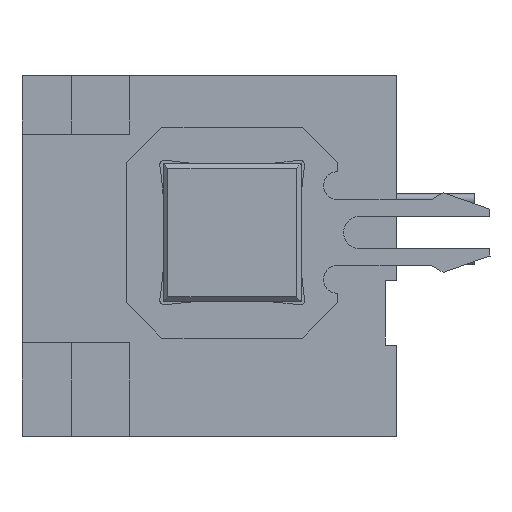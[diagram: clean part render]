
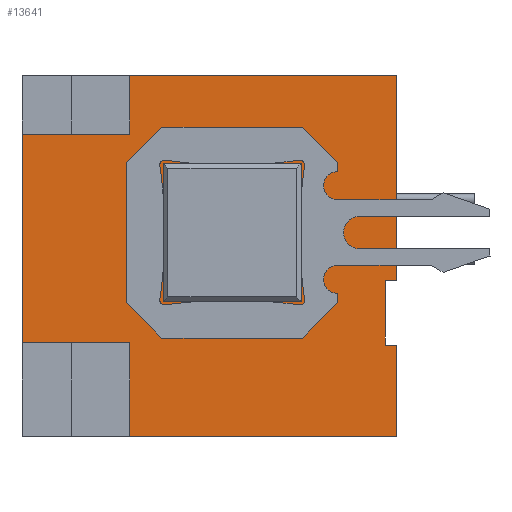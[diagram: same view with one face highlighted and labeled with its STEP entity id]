
A CAD part, left-side view. The second image highlights one B-rep face of the part: STEP entity #13641.
In plain terms, the highlighted planar face has unit normal (-1, 0, 0).
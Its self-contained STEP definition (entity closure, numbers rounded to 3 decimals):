
#40 = DIRECTION ( 'NONE',  ( 0., 0., 1. ) ) ;
#643 = DIRECTION ( 'NONE',  ( 0., 1., 0. ) ) ;
#648 = LINE ( 'NONE', #10963, #20650 ) ;
#688 = DIRECTION ( 'NONE',  ( 0., -1., 0. ) ) ;
#692 = CARTESIAN_POINT ( 'NONE',  ( -14.2, 1.975, 3.945 ) ) ;
#731 = VERTEX_POINT ( 'NONE', #20178 ) ;
#1031 = CARTESIAN_POINT ( 'NONE',  ( -14.2, -3.915, -1.945 ) ) ;
#1243 = CARTESIAN_POINT ( 'NONE',  ( -14.2, 3.4, -7.7 ) ) ;
#1359 = VERTEX_POINT ( 'NONE', #1243 ) ;
#1480 = ORIENTED_EDGE ( 'NONE', *, *, #5969, .F. ) ;
#1513 = VERTEX_POINT ( 'NONE', #15377 ) ;
#1740 = DIRECTION ( 'NONE',  ( 0., 0., 1. ) ) ;
#1865 = DIRECTION ( 'NONE',  ( 0., 0., 1. ) ) ;
#1890 = CARTESIAN_POINT ( 'NONE',  ( -14.2, 3.4, -3.7 ) ) ;
#2224 = DIRECTION ( 'NONE',  ( 0., 0., -1. ) ) ;
#2297 = VERTEX_POINT ( 'NONE', #26290 ) ;
#2396 = CARTESIAN_POINT ( 'NONE',  ( -14.2, -8., 0. ) ) ;
#2933 = LINE ( 'NONE', #2396, #24023 ) ;
#3200 = LINE ( 'NONE', #21412, #25618 ) ;
#3273 = DIRECTION ( 'NONE',  ( 0., 0., 1. ) ) ;
#3357 = LINE ( 'NONE', #13885, #6747 ) ;
#3377 = VECTOR ( 'NONE', #2224, 1000. ) ;
#3467 = EDGE_CURVE ( 'NONE', #19096, #731, #24400, .T. ) ;
#3474 = VECTOR ( 'NONE', #28197, 1000. ) ;
#3495 = LINE ( 'NONE', #22091, #16701 ) ;
#3871 = EDGE_LOOP ( 'NONE', ( #3902, #7708, #25490, #9734 ) ) ;
#3902 = ORIENTED_EDGE ( 'NONE', *, *, #3467, .T. ) ;
#4520 = CARTESIAN_POINT ( 'NONE',  ( -14.2, 1.975, 1. ) ) ;
#4812 = DIRECTION ( 'NONE',  ( 0., 1., 0. ) ) ;
#4821 = FACE_BOUND ( 'NONE', #3871, .T. ) ;
#5153 = EDGE_CURVE ( 'NONE', #24769, #12141, #3495, .T. ) ;
#5224 = VECTOR ( 'NONE', #17826, 1000. ) ;
#5384 = CARTESIAN_POINT ( 'NONE',  ( -14.2, -7.5, -1.05 ) ) ;
#5502 = CARTESIAN_POINT ( 'NONE',  ( -14.2, 3.4, 7.7 ) ) ;
#5545 = VERTEX_POINT ( 'NONE', #19291 ) ;
#5969 = EDGE_CURVE ( 'NONE', #5545, #22792, #13138, .T. ) ;
#6302 = CARTESIAN_POINT ( 'NONE',  ( -14.2, -3.915, 1. ) ) ;
#6424 = ORIENTED_EDGE ( 'NONE', *, *, #18494, .F. ) ;
#6539 = EDGE_CURVE ( 'NONE', #24769, #17950, #2933, .T. ) ;
#6632 = CARTESIAN_POINT ( 'NONE',  ( -14.2, -7.5, 0. ) ) ;
#6747 = VECTOR ( 'NONE', #3273, 1000. ) ;
#6896 = LINE ( 'NONE', #22305, #27308 ) ;
#7298 = DIRECTION ( 'NONE',  ( 0., 1., 0. ) ) ;
#7496 = LINE ( 'NONE', #9588, #24172 ) ;
#7708 = ORIENTED_EDGE ( 'NONE', *, *, #15140, .T. ) ;
#7783 = PLANE ( 'NONE',  #19110 ) ;
#7878 = CARTESIAN_POINT ( 'NONE',  ( -14.2, 8.32, 8.008 ) ) ;
#8138 = DIRECTION ( 'NONE',  ( 0., -1., 0. ) ) ;
#8441 = DIRECTION ( 'NONE',  ( 0., -1., 0. ) ) ;
#8472 = EDGE_CURVE ( 'NONE', #25409, #2297, #6896, .T. ) ;
#8482 = ORIENTED_EDGE ( 'NONE', *, *, #6539, .F. ) ;
#8525 = LINE ( 'NONE', #12983, #3474 ) ;
#8672 = VERTEX_POINT ( 'NONE', #5502 ) ;
#8795 = EDGE_CURVE ( 'NONE', #8672, #5545, #8525, .T. ) ;
#8842 = EDGE_LOOP ( 'NONE', ( #11366, #1480, #15389, #16690, #10026, #6424, #17616, #9783, #15792, #8482, #26615, #25506 ) ) ;
#9061 = DIRECTION ( 'NONE',  ( 0., 0., -1. ) ) ;
#9180 = EDGE_CURVE ( 'NONE', #1359, #25409, #23495, .T. ) ;
#9265 = CARTESIAN_POINT ( 'NONE',  ( -14.2, -7.75, -1.05 ) ) ;
#9357 = VECTOR ( 'NONE', #9061, 1000. ) ;
#9502 = VERTEX_POINT ( 'NONE', #692 ) ;
#9588 = CARTESIAN_POINT ( 'NONE',  ( -14.2, 0., 5.2 ) ) ;
#9734 = ORIENTED_EDGE ( 'NONE', *, *, #15179, .T. ) ;
#9783 = ORIENTED_EDGE ( 'NONE', *, *, #9180, .F. ) ;
#10026 = ORIENTED_EDGE ( 'NONE', *, *, #27849, .F. ) ;
#10293 = CARTESIAN_POINT ( 'NONE',  ( -14.2, -8., -1.05 ) ) ;
#10387 = EDGE_CURVE ( 'NONE', #1513, #8672, #648, .T. ) ;
#10758 = LINE ( 'NONE', #27767, #13491 ) ;
#10963 = CARTESIAN_POINT ( 'NONE',  ( -14.2, 3.4, 0. ) ) ;
#11241 = EDGE_CURVE ( 'NONE', #9502, #15343, #10758, .T. ) ;
#11366 = ORIENTED_EDGE ( 'NONE', *, *, #12251, .T. ) ;
#11656 = LINE ( 'NONE', #9265, #5224 ) ;
#12122 = LINE ( 'NONE', #6632, #23024 ) ;
#12141 = VERTEX_POINT ( 'NONE', #17726 ) ;
#12251 = EDGE_CURVE ( 'NONE', #21208, #22792, #11656, .T. ) ;
#12983 = CARTESIAN_POINT ( 'NONE',  ( -14.2, 0., 7.7 ) ) ;
#13138 = LINE ( 'NONE', #17811, #9357 ) ;
#13491 = VECTOR ( 'NONE', #8441, 1000. ) ;
#13641 = ADVANCED_FACE ( 'NONE', ( #4821, #23860 ), #7783, .F. ) ;
#13885 = CARTESIAN_POINT ( 'NONE',  ( -14.2, 8., 0. ) ) ;
#14332 = DIRECTION ( 'NONE',  ( 1., 0., 0. ) ) ;
#14651 = VECTOR ( 'NONE', #1740, 1000. ) ;
#15140 = EDGE_CURVE ( 'NONE', #731, #9502, #24761, .T. ) ;
#15179 = EDGE_CURVE ( 'NONE', #15343, #19096, #26135, .T. ) ;
#15343 = VERTEX_POINT ( 'NONE', #24912 ) ;
#15377 = CARTESIAN_POINT ( 'NONE',  ( -14.2, 3.4, 5.2 ) ) ;
#15389 = ORIENTED_EDGE ( 'NONE', *, *, #8795, .F. ) ;
#15792 = ORIENTED_EDGE ( 'NONE', *, *, #26132, .F. ) ;
#16265 = EDGE_CURVE ( 'NONE', #21208, #12141, #12122, .T. ) ;
#16690 = ORIENTED_EDGE ( 'NONE', *, *, #10387, .F. ) ;
#16701 = VECTOR ( 'NONE', #4812, 1000. ) ;
#17616 = ORIENTED_EDGE ( 'NONE', *, *, #8472, .F. ) ;
#17726 = CARTESIAN_POINT ( 'NONE',  ( -14.2, -7.5, -3.8 ) ) ;
#17811 = CARTESIAN_POINT ( 'NONE',  ( -14.2, -8., 0. ) ) ;
#17826 = DIRECTION ( 'NONE',  ( 0., -1., 0. ) ) ;
#17950 = VERTEX_POINT ( 'NONE', #20936 ) ;
#18494 = EDGE_CURVE ( 'NONE', #2297, #23355, #3357, .T. ) ;
#18635 = VECTOR ( 'NONE', #40, 1000. ) ;
#18932 = CARTESIAN_POINT ( 'NONE',  ( -14.2, 8., 5.2 ) ) ;
#19096 = VERTEX_POINT ( 'NONE', #1031 ) ;
#19110 = AXIS2_PLACEMENT_3D ( 'NONE', #7878, #14332, #8138 ) ;
#19291 = CARTESIAN_POINT ( 'NONE',  ( -14.2, -8., 7.7 ) ) ;
#20178 = CARTESIAN_POINT ( 'NONE',  ( -14.2, 1.975, -1.945 ) ) ;
#20650 = VECTOR ( 'NONE', #1865, 1000. ) ;
#20936 = CARTESIAN_POINT ( 'NONE',  ( -14.2, -8., -7.7 ) ) ;
#21208 = VERTEX_POINT ( 'NONE', #5384 ) ;
#21412 = CARTESIAN_POINT ( 'NONE',  ( -14.2, 0., -7.7 ) ) ;
#21732 = DIRECTION ( 'NONE',  ( 0., 0., -1. ) ) ;
#22091 = CARTESIAN_POINT ( 'NONE',  ( -14.2, -7.75, -3.8 ) ) ;
#22114 = CARTESIAN_POINT ( 'NONE',  ( -14.2, -0.97, -1.945 ) ) ;
#22305 = CARTESIAN_POINT ( 'NONE',  ( -14.2, 0., -3.7 ) ) ;
#22792 = VERTEX_POINT ( 'NONE', #10293 ) ;
#23024 = VECTOR ( 'NONE', #21732, 1000. ) ;
#23355 = VERTEX_POINT ( 'NONE', #18932 ) ;
#23495 = LINE ( 'NONE', #25491, #14651 ) ;
#23741 = DIRECTION ( 'NONE',  ( 0., 1., 0. ) ) ;
#23860 = FACE_OUTER_BOUND ( 'NONE', #8842, .T. ) ;
#24023 = VECTOR ( 'NONE', #24077, 1000. ) ;
#24077 = DIRECTION ( 'NONE',  ( 0., 0., -1. ) ) ;
#24172 = VECTOR ( 'NONE', #688, 1000. ) ;
#24400 = LINE ( 'NONE', #22114, #27463 ) ;
#24761 = LINE ( 'NONE', #4520, #18635 ) ;
#24769 = VERTEX_POINT ( 'NONE', #27072 ) ;
#24912 = CARTESIAN_POINT ( 'NONE',  ( -14.2, -3.915, 3.945 ) ) ;
#25409 = VERTEX_POINT ( 'NONE', #1890 ) ;
#25490 = ORIENTED_EDGE ( 'NONE', *, *, #11241, .T. ) ;
#25491 = CARTESIAN_POINT ( 'NONE',  ( -14.2, 3.4, 0. ) ) ;
#25506 = ORIENTED_EDGE ( 'NONE', *, *, #16265, .F. ) ;
#25618 = VECTOR ( 'NONE', #23741, 1000. ) ;
#26132 = EDGE_CURVE ( 'NONE', #17950, #1359, #3200, .T. ) ;
#26135 = LINE ( 'NONE', #6302, #3377 ) ;
#26290 = CARTESIAN_POINT ( 'NONE',  ( -14.2, 8., -3.7 ) ) ;
#26615 = ORIENTED_EDGE ( 'NONE', *, *, #5153, .T. ) ;
#27072 = CARTESIAN_POINT ( 'NONE',  ( -14.2, -8., -3.8 ) ) ;
#27308 = VECTOR ( 'NONE', #7298, 1000. ) ;
#27463 = VECTOR ( 'NONE', #643, 1000. ) ;
#27767 = CARTESIAN_POINT ( 'NONE',  ( -14.2, -0.97, 3.945 ) ) ;
#27849 = EDGE_CURVE ( 'NONE', #23355, #1513, #7496, .T. ) ;
#28197 = DIRECTION ( 'NONE',  ( 0., -1., 0. ) ) ;
